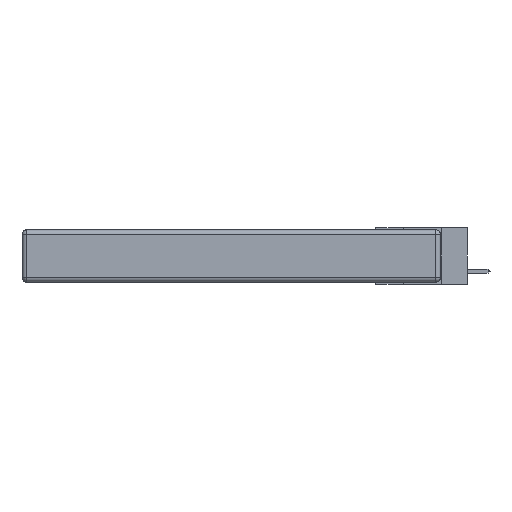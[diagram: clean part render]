
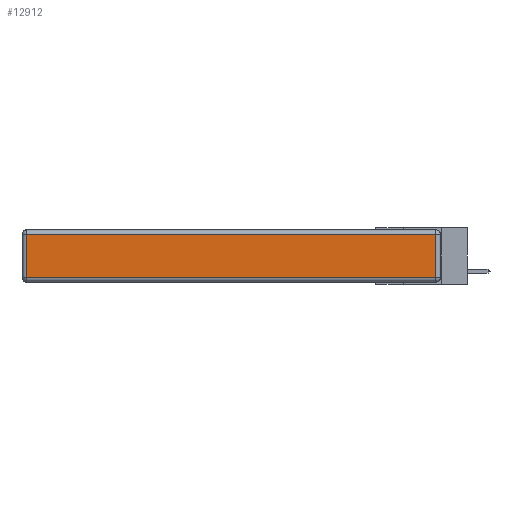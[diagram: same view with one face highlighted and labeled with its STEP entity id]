
A CAD part, left-side view. The second image highlights one B-rep face of the part: STEP entity #12912.
In plain terms, the highlighted planar face has unit normal (-1, 0, 0).
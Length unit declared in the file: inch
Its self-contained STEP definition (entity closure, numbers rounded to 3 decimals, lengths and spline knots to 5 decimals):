
#76 = PLANE ( 'NONE',  #16591 ) ;
#154 = CARTESIAN_POINT ( 'NONE',  ( 0., 0., -0.313 ) ) ;
#207 = CARTESIAN_POINT ( 'NONE',  ( 0., 0., -0.343 ) ) ;
#410 = CARTESIAN_POINT ( 'NONE',  ( 0., 0.03, -0.313 ) ) ;
#701 = LINE ( 'NONE', #154, #1498 ) ;
#917 = FACE_OUTER_BOUND ( 'NONE', #17521, .T. ) ;
#1269 = VECTOR ( 'NONE', #14293, 39.37008 ) ;
#1498 = VECTOR ( 'NONE', #18258, 39.37008 ) ;
#2093 = DIRECTION ( 'NONE',  ( 0., 0., 1. ) ) ;
#2262 = ORIENTED_EDGE ( 'NONE', *, *, #17511, .T. ) ;
#2919 = CARTESIAN_POINT ( 'NONE',  ( 0., 2.75, -0.03 ) ) ;
#4593 = ORIENTED_EDGE ( 'NONE', *, *, #14871, .T. ) ;
#5194 = ORIENTED_EDGE ( 'NONE', *, *, #9999, .T. ) ;
#5981 = VERTEX_POINT ( 'NONE', #13075 ) ;
#6448 = ORIENTED_EDGE ( 'NONE', *, *, #12379, .T. ) ;
#7416 = LINE ( 'NONE', #15612, #19133 ) ;
#7893 = VERTEX_POINT ( 'NONE', #14603 ) ;
#8833 = CARTESIAN_POINT ( 'NONE',  ( 0., 2.72, -0.03 ) ) ;
#9107 = DIRECTION ( 'NONE',  ( 0., 0., -1. ) ) ;
#9939 = DIRECTION ( 'NONE',  ( 0., 0., 1. ) ) ;
#9999 = EDGE_CURVE ( 'NONE', #11133, #5981, #7416, .T. ) ;
#10017 = LINE ( 'NONE', #2919, #1269 ) ;
#11133 = VERTEX_POINT ( 'NONE', #8833 ) ;
#12379 = EDGE_CURVE ( 'NONE', #5981, #12890, #701, .T. ) ;
#12890 = VERTEX_POINT ( 'NONE', #410 ) ;
#12904 = VECTOR ( 'NONE', #2093, 39.37008 ) ;
#12912 = ADVANCED_FACE ( 'NONE', ( #917 ), #76, .T. ) ;
#13075 = CARTESIAN_POINT ( 'NONE',  ( 0., 2.72, -0.313 ) ) ;
#14293 = DIRECTION ( 'NONE',  ( 0., 1., 0. ) ) ;
#14603 = CARTESIAN_POINT ( 'NONE',  ( 0., 0.03, -0.03 ) ) ;
#14871 = EDGE_CURVE ( 'NONE', #12890, #7893, #18543, .T. ) ;
#15238 = CARTESIAN_POINT ( 'NONE',  ( 0., 0.03, -0.343 ) ) ;
#15612 = CARTESIAN_POINT ( 'NONE',  ( 0., 2.72, -0.343 ) ) ;
#16591 = AXIS2_PLACEMENT_3D ( 'NONE', #207, #19914, #9939 ) ;
#17511 = EDGE_CURVE ( 'NONE', #7893, #11133, #10017, .T. ) ;
#17521 = EDGE_LOOP ( 'NONE', ( #6448, #4593, #2262, #5194 ) ) ;
#18258 = DIRECTION ( 'NONE',  ( 0., -1., 0. ) ) ;
#18543 = LINE ( 'NONE', #15238, #12904 ) ;
#19133 = VECTOR ( 'NONE', #9107, 39.37008 ) ;
#19914 = DIRECTION ( 'NONE',  ( -1., 0., 0. ) ) ;
